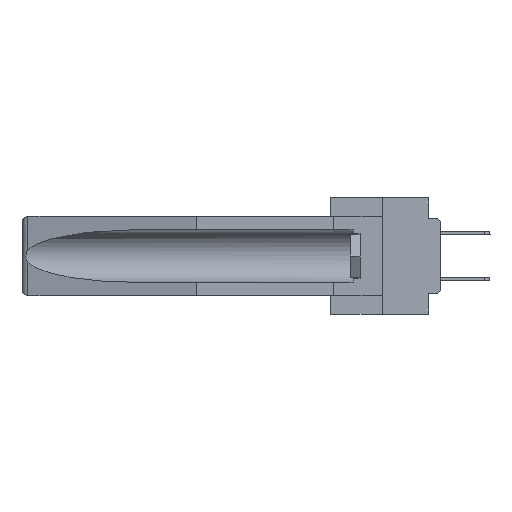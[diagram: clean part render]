
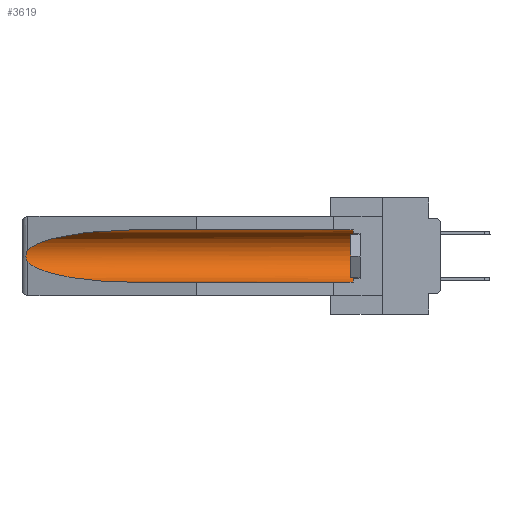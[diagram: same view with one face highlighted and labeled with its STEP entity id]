
A CAD part, left-side view. The second image highlights one B-rep face of the part: STEP entity #3619.
In plain terms, the highlighted cylindrical face has radius 2.857 mm (diameter 5.715 mm), a partial arc.
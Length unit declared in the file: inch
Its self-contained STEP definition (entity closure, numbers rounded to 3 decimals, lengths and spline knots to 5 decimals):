
#446 = DIRECTION ( 'NONE',  ( 0., -1., 0. ) ) ;
#614 = CARTESIAN_POINT ( 'NONE',  ( 0.155, 0.126, -0.1715 ) ) ;
#651 = ORIENTED_EDGE ( 'NONE', *, *, #4428, .T. ) ;
#817 = CARTESIAN_POINT ( 'NONE',  ( 0.26537, 1.52718, -0.14972 ) ) ;
#912 = DIRECTION ( 'NONE',  ( 0., 1., 0. ) ) ;
#2337 = CARTESIAN_POINT ( 'NONE',  ( 0.2675, 1.53308, -0.17534 ) ) ;
#3424 = LINE ( 'NONE', #25559, #22513 ) ;
#3619 = ADVANCED_FACE ( 'NONE', ( #32326 ), #9496, .F. ) ;
#4428 = EDGE_CURVE ( 'NONE', #10879, #14129, #26059, .T. ) ;
#4469 = CARTESIAN_POINT ( 'NONE',  ( 0.155, 1.07973, -0.059 ) ) ;
#4833 = CARTESIAN_POINT ( 'NONE',  ( 0.2673, 1.5327, -0.16383 ) ) ;
#5604 = ORIENTED_EDGE ( 'NONE', *, *, #19641, .F. ) ;
#5938 = CARTESIAN_POINT ( 'NONE',  ( 0.25451, 1.48313, -0.24835 ) ) ;
#6103 = CARTESIAN_POINT ( 'NONE',  ( 0.21114, 1.30732, -0.284 ) ) ;
#6479 = ORIENTED_EDGE ( 'NONE', *, *, #20053, .T. ) ;
#7082 = ORIENTED_EDGE ( 'NONE', *, *, #31008, .T. ) ;
#7097 =( BOUNDED_CURVE ( )  B_SPLINE_CURVE ( 3, ( #8124, #10805, #18315, #817 ),
 .UNSPECIFIED., .F., .F. ) 
 B_SPLINE_CURVE_WITH_KNOTS ( ( 4, 4 ),
 ( 4.71239, 6.08839 ),
 .UNSPECIFIED. ) 
 CURVE ( )  GEOMETRIC_REPRESENTATION_ITEM ( )  RATIONAL_B_SPLINE_CURVE ( ( 1., 0.848, 0.848, 1. ) ) 
 REPRESENTATION_ITEM ( '' )  );
#7370 = LINE ( 'NONE', #17561, #29447 ) ;
#7480 = CARTESIAN_POINT ( 'NONE',  ( 0.26655, 1.53094, -0.18657 ) ) ;
#7595 = VERTEX_POINT ( 'NONE', #10370 ) ;
#8124 = CARTESIAN_POINT ( 'NONE',  ( 0.155, 1.07973, -0.059 ) ) ;
#8263 = CARTESIAN_POINT ( 'NONE',  ( 0.26537, 1.52718, -0.19328 ) ) ;
#8513 = ORIENTED_EDGE ( 'NONE', *, *, #31184, .T. ) ;
#9496 = CYLINDRICAL_SURFACE ( 'NONE', #15745, 0.1125 ) ;
#10370 = CARTESIAN_POINT ( 'NONE',  ( 0.26537, 1.52718, -0.14972 ) ) ;
#10805 = CARTESIAN_POINT ( 'NONE',  ( 0.21114, 1.30732, -0.059 ) ) ;
#10879 = VERTEX_POINT ( 'NONE', #14143 ) ;
#11700 = CARTESIAN_POINT ( 'NONE',  ( 0.155, 0.126, -0.059 ) ) ;
#12774 = CIRCLE ( 'NONE', #28719, 0.1125 ) ;
#12813 = CARTESIAN_POINT ( 'NONE',  ( 0.26654, 1.53092, -0.15636 ) ) ;
#13274 = ORIENTED_EDGE ( 'NONE', *, *, #32356, .T. ) ;
#14129 = VERTEX_POINT ( 'NONE', #19432 ) ;
#14143 = CARTESIAN_POINT ( 'NONE',  ( 0.26537, 1.52718, -0.19328 ) ) ;
#14185 = DIRECTION ( 'NONE',  ( 0., 1., 0. ) ) ;
#14672 = CARTESIAN_POINT ( 'NONE',  ( 0.2673, 1.53269, -0.17917 ) ) ;
#14840 = CARTESIAN_POINT ( 'NONE',  ( 0.26537, 1.52718, -0.14972 ) ) ;
#15317 = CARTESIAN_POINT ( 'NONE',  ( 0.26537, 1.52718, -0.19328 ) ) ;
#15745 = AXIS2_PLACEMENT_3D ( 'NONE', #19675, #14185, #17027 ) ;
#16291 = CARTESIAN_POINT ( 'NONE',  ( 0.155, 1.07973, -0.284 ) ) ;
#17027 = DIRECTION ( 'NONE',  ( 0., 0., 1. ) ) ;
#17505 = CARTESIAN_POINT ( 'NONE',  ( 0.26597, 1.52961, -0.15275 ) ) ;
#17561 = CARTESIAN_POINT ( 'NONE',  ( 0.155, -0.30754, -0.059 ) ) ;
#17672 = VERTEX_POINT ( 'NONE', #27187 ) ;
#17860 = EDGE_LOOP ( 'NONE', ( #8513, #7082, #651, #5604, #13274, #6479 ) ) ;
#18315 = CARTESIAN_POINT ( 'NONE',  ( 0.25451, 1.48313, -0.09465 ) ) ;
#19432 = CARTESIAN_POINT ( 'NONE',  ( 0.155, 1.07973, -0.284 ) ) ;
#19641 = EDGE_CURVE ( 'NONE', #17672, #14129, #3424, .T. ) ;
#19675 = CARTESIAN_POINT ( 'NONE',  ( 0.155, -0.30754, -0.1715 ) ) ;
#20053 = EDGE_CURVE ( 'NONE', #22872, #32072, #7370, .T. ) ;
#20138 = CARTESIAN_POINT ( 'NONE',  ( 0.2675, 1.53308, -0.16763 ) ) ;
#22513 = VECTOR ( 'NONE', #912, 39.37008 ) ;
#22872 = VERTEX_POINT ( 'NONE', #11700 ) ;
#23174 = B_SPLINE_CURVE_WITH_KNOTS ( 'NONE', 3,
 ( #14840, #17505, #12813, #4833, #20138, #2337, #14672, #7480, #24970, #15317 ),
 .UNSPECIFIED., .F., .F.,
 ( 4, 2, 2, 2, 4 ),
 ( 0., 0.00029, 0.00058, 0.00087, 0.00117 ),
 .UNSPECIFIED. ) ;
#24970 = CARTESIAN_POINT ( 'NONE',  ( 0.26597, 1.5296, -0.19026 ) ) ;
#25559 = CARTESIAN_POINT ( 'NONE',  ( 0.155, -0.30754, -0.284 ) ) ;
#26059 =( BOUNDED_CURVE ( )  B_SPLINE_CURVE ( 3, ( #8263, #5938, #6103, #16291 ),
 .UNSPECIFIED., .F., .F. ) 
 B_SPLINE_CURVE_WITH_KNOTS ( ( 4, 4 ),
 ( 0.1948, 1.5708 ),
 .UNSPECIFIED. ) 
 CURVE ( )  GEOMETRIC_REPRESENTATION_ITEM ( )  RATIONAL_B_SPLINE_CURVE ( ( 1., 0.848, 0.848, 1. ) ) 
 REPRESENTATION_ITEM ( '' )  );
#26078 = DIRECTION ( 'NONE',  ( 0., 0., 1. ) ) ;
#27187 = CARTESIAN_POINT ( 'NONE',  ( 0.155, 0.126, -0.284 ) ) ;
#27699 = DIRECTION ( 'NONE',  ( 0., 1., 0. ) ) ;
#28719 = AXIS2_PLACEMENT_3D ( 'NONE', #614, #446, #26078 ) ;
#29447 = VECTOR ( 'NONE', #27699, 39.37008 ) ;
#31008 = EDGE_CURVE ( 'NONE', #7595, #10879, #23174, .T. ) ;
#31184 = EDGE_CURVE ( 'NONE', #32072, #7595, #7097, .T. ) ;
#32072 = VERTEX_POINT ( 'NONE', #4469 ) ;
#32326 = FACE_OUTER_BOUND ( 'NONE', #17860, .T. ) ;
#32356 = EDGE_CURVE ( 'NONE', #17672, #22872, #12774, .T. ) ;
